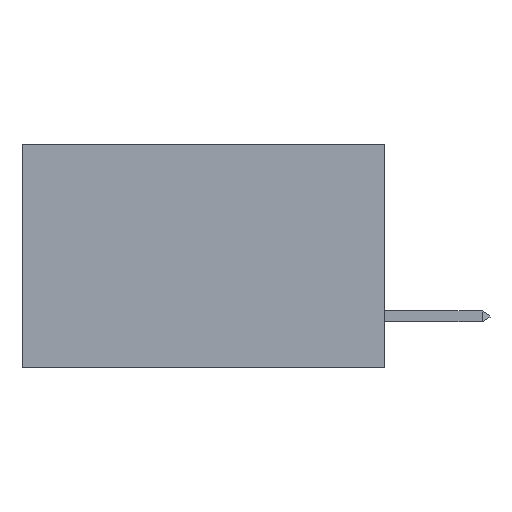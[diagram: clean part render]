
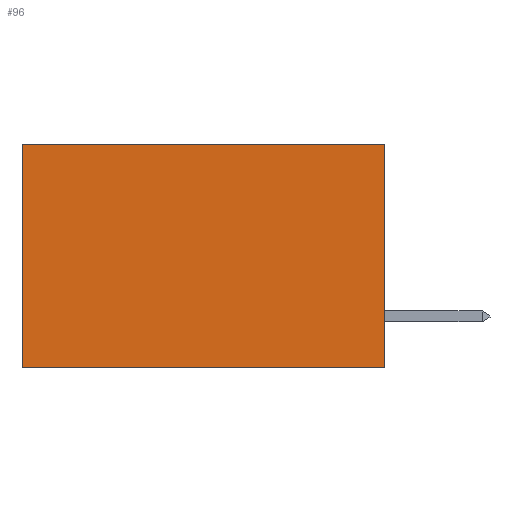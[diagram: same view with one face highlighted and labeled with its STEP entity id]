
A CAD part, left-side view. The second image highlights one B-rep face of the part: STEP entity #96.
In plain terms, the highlighted planar face has unit normal (-1, 0, 0).
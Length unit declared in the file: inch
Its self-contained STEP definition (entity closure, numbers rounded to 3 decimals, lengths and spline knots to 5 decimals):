
#96 = ADVANCED_FACE ( 'NONE', ( #12900 ), #2289, .F. ) ;
#320 = EDGE_CURVE ( 'NONE', #6983, #7915, #5152, .T. ) ;
#630 = VECTOR ( 'NONE', #3231, 39.37008 ) ;
#1367 = AXIS2_PLACEMENT_3D ( 'NONE', #13410, #9542, #3395 ) ;
#1938 = VECTOR ( 'NONE', #11281, 39.37008 ) ;
#2013 = LINE ( 'NONE', #6634, #12545 ) ;
#2247 = ORIENTED_EDGE ( 'NONE', *, *, #320, .F. ) ;
#2289 = PLANE ( 'NONE',  #1367 ) ;
#2373 = CARTESIAN_POINT ( 'NONE',  ( 0.2875, 0., 0. ) ) ;
#2748 = VERTEX_POINT ( 'NONE', #3807 ) ;
#3231 = DIRECTION ( 'NONE',  ( 0., 1., 0. ) ) ;
#3395 = DIRECTION ( 'NONE',  ( 0., 0., -1. ) ) ;
#3737 = LINE ( 'NONE', #3830, #630 ) ;
#3807 = CARTESIAN_POINT ( 'NONE',  ( 0.2875, 0.6, 0. ) ) ;
#3830 = CARTESIAN_POINT ( 'NONE',  ( 0.2875, 0., 0. ) ) ;
#4169 = EDGE_LOOP ( 'NONE', ( #10981, #10567, #2247, #11257 ) ) ;
#4806 = CARTESIAN_POINT ( 'NONE',  ( 0.2875, 0.6, -0.37 ) ) ;
#4878 = LINE ( 'NONE', #12214, #1938 ) ;
#5152 = LINE ( 'NONE', #7961, #9843 ) ;
#5988 = DIRECTION ( 'NONE',  ( 0., 0., -1. ) ) ;
#6634 = CARTESIAN_POINT ( 'NONE',  ( 0.2875, 0., -0.37 ) ) ;
#6983 = VERTEX_POINT ( 'NONE', #2373 ) ;
#7263 = EDGE_CURVE ( 'NONE', #6983, #2748, #3737, .T. ) ;
#7915 = VERTEX_POINT ( 'NONE', #10091 ) ;
#7961 = CARTESIAN_POINT ( 'NONE',  ( 0.2875, 0., 0. ) ) ;
#9542 = DIRECTION ( 'NONE',  ( 1., 0., 0. ) ) ;
#9777 = EDGE_CURVE ( 'NONE', #7915, #9885, #2013, .T. ) ;
#9843 = VECTOR ( 'NONE', #5988, 39.37008 ) ;
#9885 = VERTEX_POINT ( 'NONE', #4806 ) ;
#10091 = CARTESIAN_POINT ( 'NONE',  ( 0.2875, 0., -0.37 ) ) ;
#10567 = ORIENTED_EDGE ( 'NONE', *, *, #9777, .F. ) ;
#10573 = DIRECTION ( 'NONE',  ( 0., 1., 0. ) ) ;
#10981 = ORIENTED_EDGE ( 'NONE', *, *, #11865, .T. ) ;
#11257 = ORIENTED_EDGE ( 'NONE', *, *, #7263, .T. ) ;
#11281 = DIRECTION ( 'NONE',  ( 0., 0., -1. ) ) ;
#11865 = EDGE_CURVE ( 'NONE', #2748, #9885, #4878, .T. ) ;
#12214 = CARTESIAN_POINT ( 'NONE',  ( 0.2875, 0.6, 0. ) ) ;
#12545 = VECTOR ( 'NONE', #10573, 39.37008 ) ;
#12900 = FACE_OUTER_BOUND ( 'NONE', #4169, .T. ) ;
#13410 = CARTESIAN_POINT ( 'NONE',  ( 0.2875, 0., 0. ) ) ;
